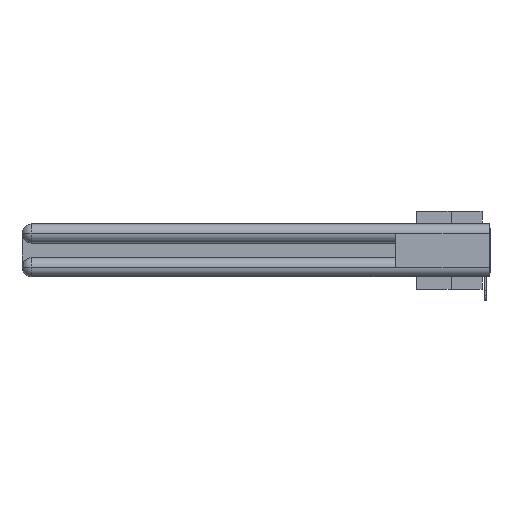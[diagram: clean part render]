
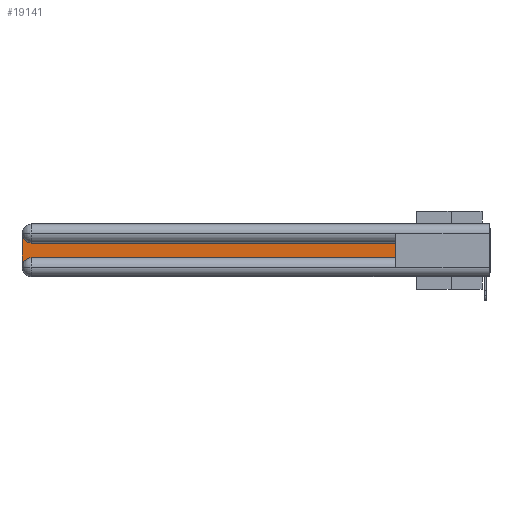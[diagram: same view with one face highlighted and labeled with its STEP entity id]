
A CAD part, left-side view. The second image highlights one B-rep face of the part: STEP entity #19141.
In plain terms, the highlighted planar face has unit normal (-1, 0, 0).
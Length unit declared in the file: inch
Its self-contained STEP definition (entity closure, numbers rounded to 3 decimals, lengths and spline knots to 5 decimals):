
#237 = CARTESIAN_POINT ( 'NONE',  ( 0.075, 2.94, -0.0625 ) ) ;
#444 = EDGE_CURVE ( 'NONE', #27515, #18777, #11140, .T. ) ;
#2607 = FACE_OUTER_BOUND ( 'NONE', #13644, .T. ) ;
#2764 = AXIS2_PLACEMENT_3D ( 'NONE', #3162, #2957, #7568 ) ;
#2957 = DIRECTION ( 'NONE',  ( 1., 0., 0. ) ) ;
#3162 = CARTESIAN_POINT ( 'NONE',  ( 0.075, 3., -0.1225 ) ) ;
#3718 = CIRCLE ( 'NONE', #8580, 0.06 ) ;
#4179 = CARTESIAN_POINT ( 'NONE',  ( 0.075, 3., -0.0625 ) ) ;
#4913 = EDGE_CURVE ( 'NONE', #27669, #11931, #23784, .T. ) ;
#5448 = LINE ( 'NONE', #7620, #13216 ) ;
#5504 = CARTESIAN_POINT ( 'NONE',  ( 0.075, 2.94, -0.1225 ) ) ;
#6644 = ORIENTED_EDGE ( 'NONE', *, *, #27661, .T. ) ;
#7314 = EDGE_CURVE ( 'NONE', #11931, #18182, #8043, .T. ) ;
#7568 = DIRECTION ( 'NONE',  ( 0., 0., -1. ) ) ;
#7582 = CARTESIAN_POINT ( 'NONE',  ( 0.075, 0.6, -0.2175 ) ) ;
#7620 = CARTESIAN_POINT ( 'NONE',  ( 0.075, 0.6, -0.2175 ) ) ;
#7939 = CARTESIAN_POINT ( 'NONE',  ( 0.075, 0.6, -0.1225 ) ) ;
#8043 = LINE ( 'NONE', #13067, #10256 ) ;
#8550 = DIRECTION ( 'NONE',  ( 0., 1., 0. ) ) ;
#8580 = AXIS2_PLACEMENT_3D ( 'NONE', #25914, #18849, #28236 ) ;
#9666 = CARTESIAN_POINT ( 'NONE',  ( 0.075, 0.6, -0.2175 ) ) ;
#10256 = VECTOR ( 'NONE', #15135, 39.37008 ) ;
#11140 = LINE ( 'NONE', #7582, #25981 ) ;
#11323 = CARTESIAN_POINT ( 'NONE',  ( 0.075, 3., -0.2775 ) ) ;
#11931 = VERTEX_POINT ( 'NONE', #4179 ) ;
#12036 = EDGE_CURVE ( 'NONE', #18182, #17173, #3718, .T. ) ;
#12192 = AXIS2_PLACEMENT_3D ( 'NONE', #237, #19192, #27094 ) ;
#12321 = ORIENTED_EDGE ( 'NONE', *, *, #22884, .T. ) ;
#13067 = CARTESIAN_POINT ( 'NONE',  ( 0.075, 3., -0.2175 ) ) ;
#13216 = VECTOR ( 'NONE', #26571, 39.37008 ) ;
#13644 = EDGE_LOOP ( 'NONE', ( #12321, #26781, #27079, #23291, #6644, #24687 ) ) ;
#15135 = DIRECTION ( 'NONE',  ( 0., 0., -1. ) ) ;
#17154 = PLANE ( 'NONE',  #2764 ) ;
#17173 = VERTEX_POINT ( 'NONE', #26045 ) ;
#18182 = VERTEX_POINT ( 'NONE', #11323 ) ;
#18321 = VECTOR ( 'NONE', #8550, 39.37008 ) ;
#18777 = VERTEX_POINT ( 'NONE', #22536 ) ;
#18849 = DIRECTION ( 'NONE',  ( 1., 0., 0. ) ) ;
#19141 = ADVANCED_FACE ( 'NONE', ( #2607 ), #17154, .F. ) ;
#19192 = DIRECTION ( 'NONE',  ( 1., 0., 0. ) ) ;
#21708 = DIRECTION ( 'NONE',  ( 0., 0., 1. ) ) ;
#22536 = CARTESIAN_POINT ( 'NONE',  ( 0.075, 0.6, -0.1225 ) ) ;
#22884 = EDGE_CURVE ( 'NONE', #18777, #27669, #24618, .T. ) ;
#23291 = ORIENTED_EDGE ( 'NONE', *, *, #12036, .T. ) ;
#23784 = CIRCLE ( 'NONE', #12192, 0.06 ) ;
#24618 = LINE ( 'NONE', #7939, #18321 ) ;
#24687 = ORIENTED_EDGE ( 'NONE', *, *, #444, .T. ) ;
#25914 = CARTESIAN_POINT ( 'NONE',  ( 0.075, 2.94, -0.2775 ) ) ;
#25981 = VECTOR ( 'NONE', #21708, 39.37008 ) ;
#26045 = CARTESIAN_POINT ( 'NONE',  ( 0.075, 2.94, -0.2175 ) ) ;
#26571 = DIRECTION ( 'NONE',  ( 0., -1., 0. ) ) ;
#26781 = ORIENTED_EDGE ( 'NONE', *, *, #4913, .T. ) ;
#27079 = ORIENTED_EDGE ( 'NONE', *, *, #7314, .T. ) ;
#27094 = DIRECTION ( 'NONE',  ( 0., 0., -1. ) ) ;
#27515 = VERTEX_POINT ( 'NONE', #9666 ) ;
#27661 = EDGE_CURVE ( 'NONE', #17173, #27515, #5448, .T. ) ;
#27669 = VERTEX_POINT ( 'NONE', #5504 ) ;
#28236 = DIRECTION ( 'NONE',  ( 0., 0., -1. ) ) ;
